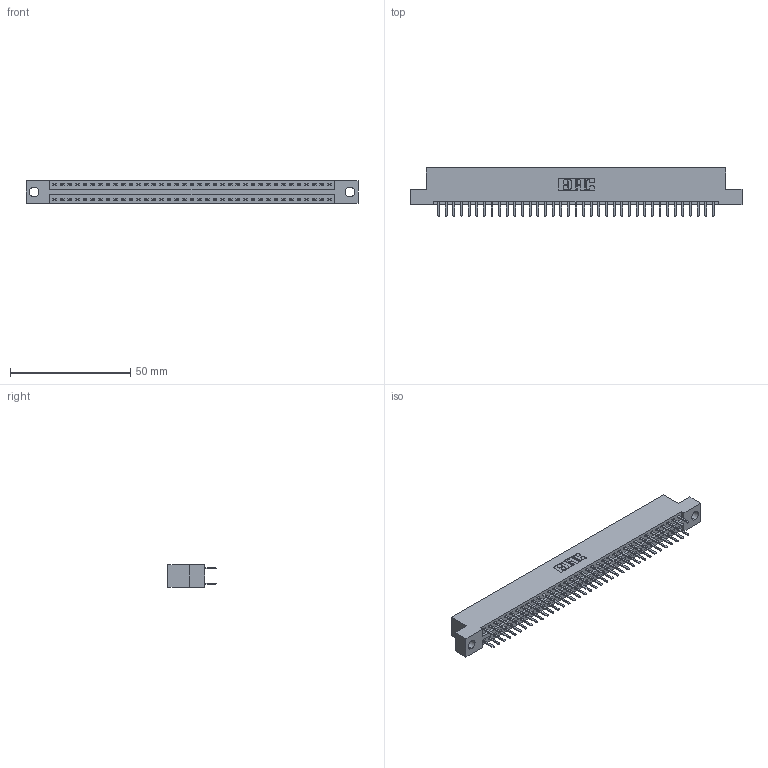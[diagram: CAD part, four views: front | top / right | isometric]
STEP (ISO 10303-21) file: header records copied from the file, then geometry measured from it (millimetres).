
FILE_DESCRIPTION (( 'STEP AP203' ), '1' );
FILE_NAME ('346-074-520-204.STEP', '2022-05-25T01:37:46', ( '' ), ( '' ), 'SwSTEP 2.0', 'SolidWorks 2020', '' );
FILE_SCHEMA (( 'CONFIG_CONTROL_DESIGN' ));
Length unit declared in the file: inch
Products named in the file (3): 346 Part_Flush Mounting Lugs - 0.156 Dia-TH; 346-074-520-204; 345-292-001_345-293-120
Assembly tree (75 placements, depth 2):
  346-074-520-204
    346 Part_Flush Mounting Lugs - 0.156 Dia-TH
    345-292-001_345-293-120  x74
Bounding box: 138.05 x 20.02 x 9.4 mm (x, y, z)
Volume: 13284.2 mm3; surface area: 17953.1 mm2
Topology: 75 solids, 75 shells, 4280 faces, 12427 edges, 8086 vertices
Faces by surface type: plane 2828, cylinder 1452
Entity records: 25353 total; most frequent: CARTESIAN_POINT 4202, ORIENTED_EDGE 4122, DIRECTION 3741, EDGE_CURVE 2061, VECTOR 1777, LINE 1777, VERTEX_POINT 1370, AXIS2_PLACEMENT_3D 982
